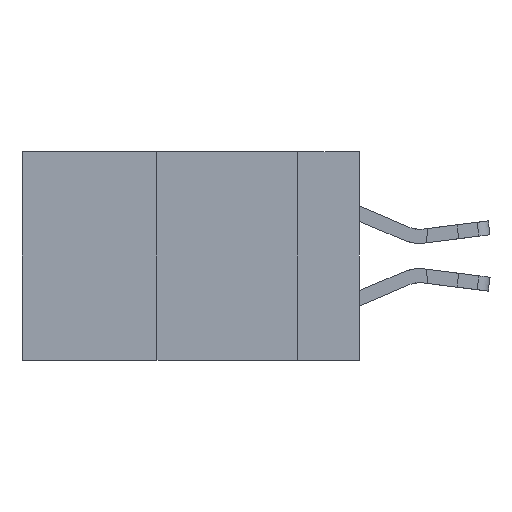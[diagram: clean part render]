
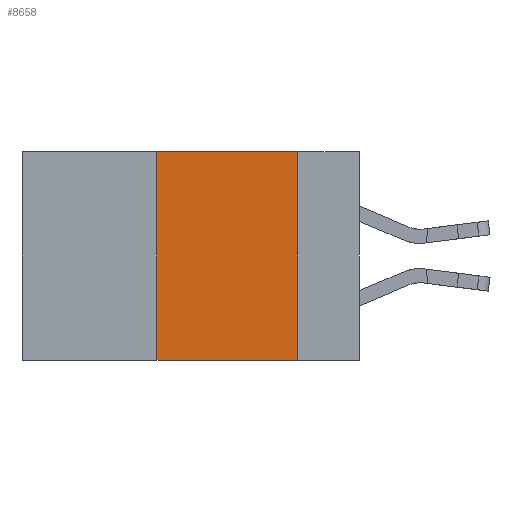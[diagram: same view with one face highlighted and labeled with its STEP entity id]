
A CAD part, left-side view. The second image highlights one B-rep face of the part: STEP entity #8658.
In plain terms, the highlighted planar face has unit normal (-1, 0, 0).
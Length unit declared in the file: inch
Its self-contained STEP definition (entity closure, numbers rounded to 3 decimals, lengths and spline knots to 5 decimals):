
#493 = AXIS2_PLACEMENT_3D ( 'NONE', #9254, #14140, #8967 ) ;
#739 = VECTOR ( 'NONE', #19161, 39.37008 ) ;
#1056 = VECTOR ( 'NONE', #6224, 39.37008 ) ;
#1143 = EDGE_CURVE ( 'NONE', #17349, #8585, #13950, .T. ) ;
#3357 = CARTESIAN_POINT ( 'NONE',  ( 0., 0.6, 0. ) ) ;
#3497 = DIRECTION ( 'NONE',  ( 0., -1., 0. ) ) ;
#4017 = EDGE_CURVE ( 'NONE', #16384, #8585, #8574, .T. ) ;
#4546 = VECTOR ( 'NONE', #3497, 39.37008 ) ;
#4604 = CARTESIAN_POINT ( 'NONE',  ( 0., 0.6, -0.37 ) ) ;
#5785 = LINE ( 'NONE', #3357, #18243 ) ;
#6224 = DIRECTION ( 'NONE',  ( 0., 0., 1. ) ) ;
#6549 = ORIENTED_EDGE ( 'NONE', *, *, #4017, .T. ) ;
#6842 = CARTESIAN_POINT ( 'NONE',  ( 0., 0.36, 0. ) ) ;
#8574 = LINE ( 'NONE', #4604, #4546 ) ;
#8585 = VERTEX_POINT ( 'NONE', #20148 ) ;
#8658 = ADVANCED_FACE ( 'NONE', ( #11189 ), #12503, .F. ) ;
#8967 = DIRECTION ( 'NONE',  ( 0., 0., -1. ) ) ;
#9254 = CARTESIAN_POINT ( 'NONE',  ( 0., 0.6, 0. ) ) ;
#11189 = FACE_OUTER_BOUND ( 'NONE', #12689, .T. ) ;
#12090 = CARTESIAN_POINT ( 'NONE',  ( 0., 0.36, -0.37 ) ) ;
#12503 = PLANE ( 'NONE',  #493 ) ;
#12689 = EDGE_LOOP ( 'NONE', ( #18556, #15716, #18506, #6549 ) ) ;
#12802 = DIRECTION ( 'NONE',  ( 0., -1., 0. ) ) ;
#13950 = LINE ( 'NONE', #14296, #739 ) ;
#14140 = DIRECTION ( 'NONE',  ( 1., 0., 0. ) ) ;
#14296 = CARTESIAN_POINT ( 'NONE',  ( 0., 0.11, 0. ) ) ;
#15201 = EDGE_CURVE ( 'NONE', #16384, #17019, #19138, .T. ) ;
#15716 = ORIENTED_EDGE ( 'NONE', *, *, #16846, .F. ) ;
#15920 = CARTESIAN_POINT ( 'NONE',  ( 0., 0.36, 0. ) ) ;
#16384 = VERTEX_POINT ( 'NONE', #12090 ) ;
#16846 = EDGE_CURVE ( 'NONE', #17019, #17349, #5785, .T. ) ;
#17019 = VERTEX_POINT ( 'NONE', #6842 ) ;
#17349 = VERTEX_POINT ( 'NONE', #17773 ) ;
#17773 = CARTESIAN_POINT ( 'NONE',  ( 0., 0.11, 0. ) ) ;
#18243 = VECTOR ( 'NONE', #12802, 39.37008 ) ;
#18506 = ORIENTED_EDGE ( 'NONE', *, *, #15201, .F. ) ;
#18556 = ORIENTED_EDGE ( 'NONE', *, *, #1143, .F. ) ;
#19138 = LINE ( 'NONE', #15920, #1056 ) ;
#19161 = DIRECTION ( 'NONE',  ( 0., 0., -1. ) ) ;
#20148 = CARTESIAN_POINT ( 'NONE',  ( 0., 0.11, -0.37 ) ) ;
